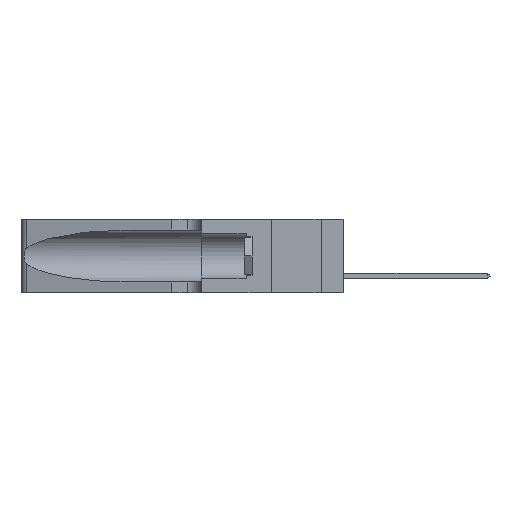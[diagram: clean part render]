
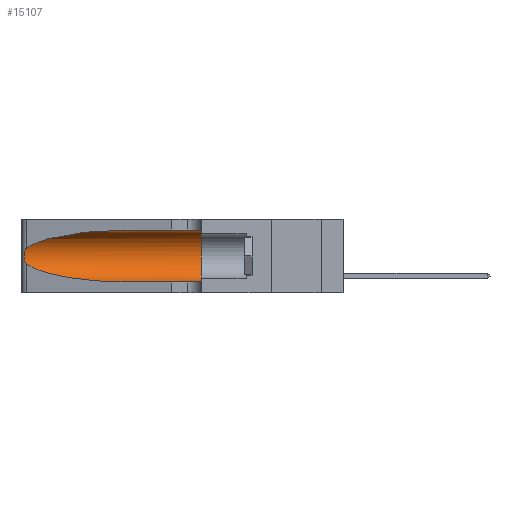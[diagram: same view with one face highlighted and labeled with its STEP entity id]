
A CAD part, left-side view. The second image highlights one B-rep face of the part: STEP entity #15107.
In plain terms, the highlighted cylindrical face has radius 3.308 mm (diameter 6.617 mm), a partial arc.
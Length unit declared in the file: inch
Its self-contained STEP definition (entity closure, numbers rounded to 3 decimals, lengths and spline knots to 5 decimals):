
#276 = ORIENTED_EDGE ( 'NONE', *, *, #11408, .T. ) ;
#715 = CARTESIAN_POINT ( 'NONE',  ( 0.18966, 0.96281, 0.05475 ) ) ;
#1026 = CARTESIAN_POINT ( 'NONE',  ( 0.26075, 1.23896, 0.178 ) ) ;
#1114 = CARTESIAN_POINT ( 'NONE',  ( 0.1305, 0.72297, 0.05475 ) ) ;
#3613 = CARTESIAN_POINT ( 'NONE',  ( 0.25639, 1.23184, 0.21858 ) ) ;
#3707 = CARTESIAN_POINT ( 'NONE',  ( 0.26075, 1.23896, 0.19203 ) ) ;
#4296 = CARTESIAN_POINT ( 'NONE',  ( 0.1305, 1.61858, 0.31525 ) ) ;
#5021 = CARTESIAN_POINT ( 'NONE',  ( 0.25487, 1.22718, 0.14631 ) ) ;
#5259 = EDGE_CURVE ( 'NONE', #32810, #9105, #27692, .T. ) ;
#6477 = CARTESIAN_POINT ( 'NONE',  ( 0.25789, 1.23486, 0.15765 ) ) ;
#6851 = CYLINDRICAL_SURFACE ( 'NONE', #37986, 0.13025 ) ;
#7408 = DIRECTION ( 'NONE',  ( 0., -1., 0. ) ) ;
#7550 = CARTESIAN_POINT ( 'NONE',  ( 0.25487, 1.22718, 0.22369 ) ) ;
#8754 = CARTESIAN_POINT ( 'NONE',  ( 0.25487, 1.22718, 0.14631 ) ) ;
#9105 = VERTEX_POINT ( 'NONE', #5021 ) ;
#9128 = CARTESIAN_POINT ( 'NONE',  ( 0.1305, 0.72297, 0.05475 ) ) ;
#9189 = CARTESIAN_POINT ( 'NONE',  ( 0.1305, 0.35, 0.31525 ) ) ;
#9326 = CARTESIAN_POINT ( 'NONE',  ( 0.2373, 1.15595, 0.08982 ) ) ;
#9867 = DIRECTION ( 'NONE',  ( 0., -1., 0. ) ) ;
#10276 = AXIS2_PLACEMENT_3D ( 'NONE', #15247, #37852, #12182 ) ;
#10859 = CARTESIAN_POINT ( 'NONE',  ( 0.26018, 1.23835, 0.19895 ) ) ;
#11408 = EDGE_CURVE ( 'NONE', #9105, #33614, #14491, .T. ) ;
#12165 = CARTESIAN_POINT ( 'NONE',  ( 0.25856, 1.23593, 0.16098 ) ) ;
#12182 = DIRECTION ( 'NONE',  ( 0., 0., 1. ) ) ;
#12545 = CARTESIAN_POINT ( 'NONE',  ( 0.25555, 1.22993, 0.14849 ) ) ;
#14491 =( BOUNDED_CURVE ( )  B_SPLINE_CURVE ( 3, ( #8754, #9326, #715, #1114 ),
 .UNSPECIFIED., .F., .F. ) 
 B_SPLINE_CURVE_WITH_KNOTS ( ( 4, 4 ),
 ( 3.44316, 4.71239 ),
 .UNSPECIFIED. ) 
 CURVE ( )  GEOMETRIC_REPRESENTATION_ITEM ( )  RATIONAL_B_SPLINE_CURVE ( ( 1., 0.87, 0.87, 1. ) ) 
 REPRESENTATION_ITEM ( '' )  );
#15107 = ADVANCED_FACE ( 'NONE', ( #23026 ), #6851, .F. ) ;
#15247 = CARTESIAN_POINT ( 'NONE',  ( 0.1305, 0.35, 0.185 ) ) ;
#15724 = CARTESIAN_POINT ( 'NONE',  ( 0.2373, 1.15595, 0.28018 ) ) ;
#16298 = EDGE_LOOP ( 'NONE', ( #17988, #41151, #276, #21676, #41215, #21503 ) ) ;
#17988 = ORIENTED_EDGE ( 'NONE', *, *, #34703, .T. ) ;
#18235 = DIRECTION ( 'NONE',  ( 0., -1., 0. ) ) ;
#18917 = VECTOR ( 'NONE', #18235, 39.37008 ) ;
#19105 = EDGE_CURVE ( 'NONE', #33614, #22684, #28025, .T. ) ;
#19109 = CARTESIAN_POINT ( 'NONE',  ( 0.25487, 1.22718, 0.22369 ) ) ;
#19703 = CARTESIAN_POINT ( 'NONE',  ( 0.25487, 1.22718, 0.22369 ) ) ;
#20589 = CARTESIAN_POINT ( 'NONE',  ( 0.26017, 1.23833, 0.17102 ) ) ;
#20851 = CARTESIAN_POINT ( 'NONE',  ( 0.1305, 0.35, 0.05475 ) ) ;
#21038 = DIRECTION ( 'NONE',  ( 0., 0., -1. ) ) ;
#21503 = ORIENTED_EDGE ( 'NONE', *, *, #34907, .F. ) ;
#21676 = ORIENTED_EDGE ( 'NONE', *, *, #19105, .T. ) ;
#21729 = CARTESIAN_POINT ( 'NONE',  ( 0.25787, 1.23484, 0.2124 ) ) ;
#22684 = VERTEX_POINT ( 'NONE', #20851 ) ;
#23026 = FACE_OUTER_BOUND ( 'NONE', #16298, .T. ) ;
#23078 = CIRCLE ( 'NONE', #10276, 0.13025 ) ;
#23292 = VERTEX_POINT ( 'NONE', #9189 ) ;
#24600 = CARTESIAN_POINT ( 'NONE',  ( 0.1305, 1.61858, 0.05475 ) ) ;
#25079 = CARTESIAN_POINT ( 'NONE',  ( 0.1305, 1.61858, 0.185 ) ) ;
#25539 = CARTESIAN_POINT ( 'NONE',  ( 0.25854, 1.2359, 0.20912 ) ) ;
#25660 = LINE ( 'NONE', #4296, #39814 ) ;
#27112 = CARTESIAN_POINT ( 'NONE',  ( 0.1305, 0.72297, 0.31525 ) ) ;
#27692 = B_SPLINE_CURVE_WITH_KNOTS ( 'NONE', 3,
 ( #19703, #40718, #3613, #21729, #25539, #10859, #3707, #1026, #20589, #12165, #6477, #39399, #12545, #32720 ),
 .UNSPECIFIED., .F., .F.,
 ( 4, 2, 2, 2, 2, 2, 4 ),
 ( 0., 0.00027, 0.00053, 0.00107, 0.0016, 0.00187, 0.00214 ),
 .UNSPECIFIED. ) ;
#28025 = LINE ( 'NONE', #24600, #18917 ) ;
#28472 = CARTESIAN_POINT ( 'NONE',  ( 0.18966, 0.96281, 0.31525 ) ) ;
#28673 = VERTEX_POINT ( 'NONE', #27112 ) ;
#32720 = CARTESIAN_POINT ( 'NONE',  ( 0.25487, 1.22718, 0.14631 ) ) ;
#32810 = VERTEX_POINT ( 'NONE', #7550 ) ;
#33614 = VERTEX_POINT ( 'NONE', #9128 ) ;
#34703 = EDGE_CURVE ( 'NONE', #28673, #32810, #37779, .T. ) ;
#34832 = CARTESIAN_POINT ( 'NONE',  ( 0.1305, 0.72297, 0.31525 ) ) ;
#34907 = EDGE_CURVE ( 'NONE', #28673, #23292, #25660, .T. ) ;
#37779 =( BOUNDED_CURVE ( )  B_SPLINE_CURVE ( 3, ( #34832, #28472, #15724, #19109 ),
 .UNSPECIFIED., .F., .F. ) 
 B_SPLINE_CURVE_WITH_KNOTS ( ( 4, 4 ),
 ( 1.5708, 2.84003 ),
 .UNSPECIFIED. ) 
 CURVE ( )  GEOMETRIC_REPRESENTATION_ITEM ( )  RATIONAL_B_SPLINE_CURVE ( ( 1., 0.87, 0.87, 1. ) ) 
 REPRESENTATION_ITEM ( '' )  );
#37852 = DIRECTION ( 'NONE',  ( 0., 1., 0. ) ) ;
#37986 = AXIS2_PLACEMENT_3D ( 'NONE', #25079, #9867, #21038 ) ;
#39399 = CARTESIAN_POINT ( 'NONE',  ( 0.25639, 1.23186, 0.15144 ) ) ;
#39814 = VECTOR ( 'NONE', #7408, 39.37008 ) ;
#40718 = CARTESIAN_POINT ( 'NONE',  ( 0.25555, 1.22994, 0.2215 ) ) ;
#41151 = ORIENTED_EDGE ( 'NONE', *, *, #5259, .T. ) ;
#41215 = ORIENTED_EDGE ( 'NONE', *, *, #41229, .F. ) ;
#41229 = EDGE_CURVE ( 'NONE', #23292, #22684, #23078, .T. ) ;
